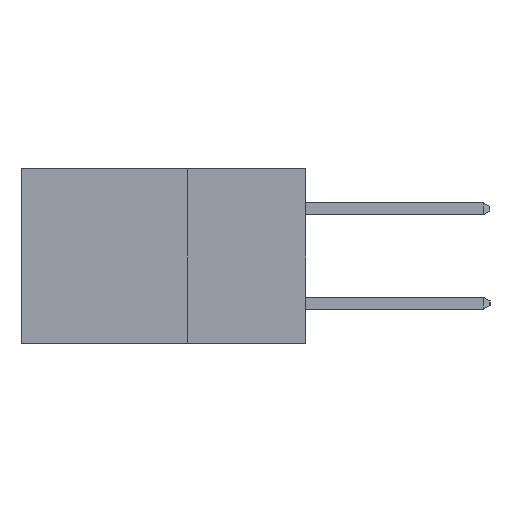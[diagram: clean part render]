
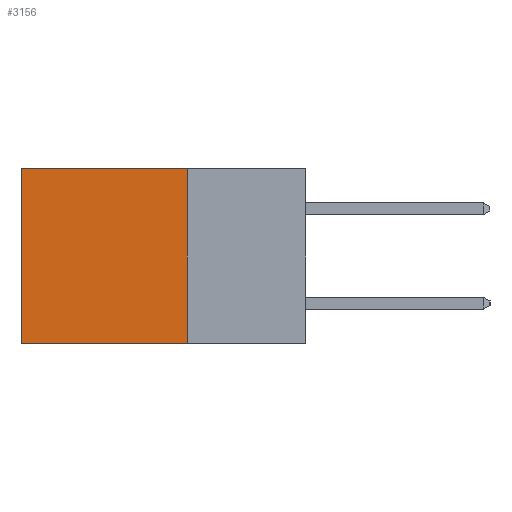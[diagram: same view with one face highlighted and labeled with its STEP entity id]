
A CAD part, left-side view. The second image highlights one B-rep face of the part: STEP entity #3156.
In plain terms, the highlighted planar face has unit normal (-1, 0, 0).
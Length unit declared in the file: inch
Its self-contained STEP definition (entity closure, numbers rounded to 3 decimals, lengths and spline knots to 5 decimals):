
#46 = CARTESIAN_POINT ( 'NONE',  ( 0.2615, 0.25, 0. ) ) ;
#260 = VECTOR ( 'NONE', #306, 39.37008 ) ;
#306 = DIRECTION ( 'NONE',  ( 0., 1., 0. ) ) ;
#515 = LINE ( 'NONE', #13363, #5994 ) ;
#806 = CARTESIAN_POINT ( 'NONE',  ( 0.2615, 0.25, 0. ) ) ;
#877 = LINE ( 'NONE', #806, #260 ) ;
#1096 = CARTESIAN_POINT ( 'NONE',  ( 0.2615, 0.6, -0.37 ) ) ;
#1292 = ORIENTED_EDGE ( 'NONE', *, *, #5233, .F. ) ;
#1390 = EDGE_LOOP ( 'NONE', ( #5417, #5759, #1292, #10285 ) ) ;
#2465 = VERTEX_POINT ( 'NONE', #8462 ) ;
#2530 = VERTEX_POINT ( 'NONE', #7653 ) ;
#3028 = EDGE_CURVE ( 'NONE', #2465, #2530, #515, .T. ) ;
#3048 = LINE ( 'NONE', #3397, #4074 ) ;
#3156 = ADVANCED_FACE ( 'NONE', ( #13340 ), #10882, .F. ) ;
#3291 = LINE ( 'NONE', #1096, #11512 ) ;
#3336 = VERTEX_POINT ( 'NONE', #6992 ) ;
#3397 = CARTESIAN_POINT ( 'NONE',  ( 0.2615, 0.25, -0.37 ) ) ;
#3905 = VERTEX_POINT ( 'NONE', #46 ) ;
#4074 = VECTOR ( 'NONE', #11952, 39.37008 ) ;
#5233 = EDGE_CURVE ( 'NONE', #3905, #2465, #3048, .T. ) ;
#5417 = ORIENTED_EDGE ( 'NONE', *, *, #8498, .T. ) ;
#5759 = ORIENTED_EDGE ( 'NONE', *, *, #3028, .F. ) ;
#5994 = VECTOR ( 'NONE', #13055, 39.37008 ) ;
#6992 = CARTESIAN_POINT ( 'NONE',  ( 0.2615, 0.6, 0. ) ) ;
#7559 = DIRECTION ( 'NONE',  ( 0., 0., -1. ) ) ;
#7653 = CARTESIAN_POINT ( 'NONE',  ( 0.2615, 0.6, -0.37 ) ) ;
#8462 = CARTESIAN_POINT ( 'NONE',  ( 0.2615, 0.25, -0.37 ) ) ;
#8498 = EDGE_CURVE ( 'NONE', #3336, #2530, #3291, .T. ) ;
#10285 = ORIENTED_EDGE ( 'NONE', *, *, #13628, .T. ) ;
#10852 = DIRECTION ( 'NONE',  ( 0., 0., -1. ) ) ;
#10868 = DIRECTION ( 'NONE',  ( 1., 0., 0. ) ) ;
#10882 = PLANE ( 'NONE',  #11385 ) ;
#11068 = CARTESIAN_POINT ( 'NONE',  ( 0.2615, 0.25, -0.37 ) ) ;
#11385 = AXIS2_PLACEMENT_3D ( 'NONE', #11068, #10868, #10852 ) ;
#11512 = VECTOR ( 'NONE', #7559, 39.37008 ) ;
#11952 = DIRECTION ( 'NONE',  ( 0., 0., -1. ) ) ;
#13055 = DIRECTION ( 'NONE',  ( 0., 1., 0. ) ) ;
#13340 = FACE_OUTER_BOUND ( 'NONE', #1390, .T. ) ;
#13363 = CARTESIAN_POINT ( 'NONE',  ( 0.2615, 0.25, -0.37 ) ) ;
#13628 = EDGE_CURVE ( 'NONE', #3905, #3336, #877, .T. ) ;
